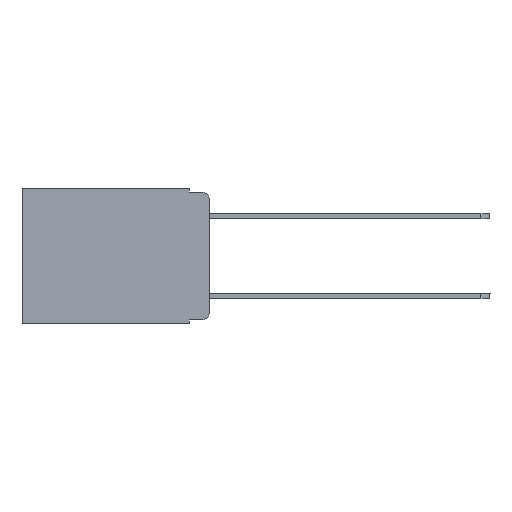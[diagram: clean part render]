
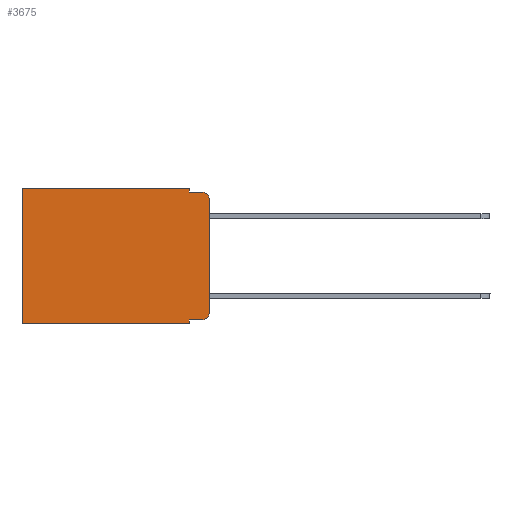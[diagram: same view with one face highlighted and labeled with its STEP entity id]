
A CAD part, left-side view. The second image highlights one B-rep face of the part: STEP entity #3675.
In plain terms, the highlighted planar face has unit normal (-1, 0, 0).
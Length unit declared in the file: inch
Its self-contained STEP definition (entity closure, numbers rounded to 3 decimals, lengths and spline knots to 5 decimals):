
#156 = EDGE_CURVE ( 'NONE', #4196, #10842, #6852, .T. ) ;
#284 = ORIENTED_EDGE ( 'NONE', *, *, #156, .T. ) ;
#360 = ORIENTED_EDGE ( 'NONE', *, *, #9546, .F. ) ;
#368 = VECTOR ( 'NONE', #1976, 39.37008 ) ;
#639 = DIRECTION ( 'NONE',  ( 0., -1., 0. ) ) ;
#705 = CARTESIAN_POINT ( 'NONE',  ( 0.298, 0., -0.03 ) ) ;
#710 = EDGE_CURVE ( 'NONE', #13267, #7853, #1727, .T. ) ;
#853 = VERTEX_POINT ( 'NONE', #5528 ) ;
#1153 = CARTESIAN_POINT ( 'NONE',  ( 0.298, 0.473, -0.343 ) ) ;
#1529 = VECTOR ( 'NONE', #7250, 39.37008 ) ;
#1727 = LINE ( 'NONE', #10578, #11859 ) ;
#1976 = DIRECTION ( 'NONE',  ( 0., 1., 0. ) ) ;
#2025 = CIRCLE ( 'NONE', #10658, 0.02 ) ;
#2625 = VERTEX_POINT ( 'NONE', #4624 ) ;
#2650 = CARTESIAN_POINT ( 'NONE',  ( 0.298, 0.02, -0.01 ) ) ;
#2816 = LINE ( 'NONE', #3873, #1529 ) ;
#2845 = DIRECTION ( 'NONE',  ( 0., 0., -1. ) ) ;
#2899 = DIRECTION ( 'NONE',  ( 0., 0., -1. ) ) ;
#2905 = CARTESIAN_POINT ( 'NONE',  ( 0.298, 0.051, -0.333 ) ) ;
#3022 = EDGE_CURVE ( 'NONE', #13267, #6196, #7514, .T. ) ;
#3092 = DIRECTION ( 'NONE',  ( -1., 0., 0. ) ) ;
#3662 = LINE ( 'NONE', #9221, #3977 ) ;
#3675 = ADVANCED_FACE ( 'NONE', ( #10889 ), #4963, .F. ) ;
#3873 = CARTESIAN_POINT ( 'NONE',  ( 0.298, 0.051, 0. ) ) ;
#3977 = VECTOR ( 'NONE', #13740, 39.37008 ) ;
#3985 = CARTESIAN_POINT ( 'NONE',  ( 0.298, 0., 0. ) ) ;
#4196 = VERTEX_POINT ( 'NONE', #2905 ) ;
#4624 = CARTESIAN_POINT ( 'NONE',  ( 0.298, 0.473, 0. ) ) ;
#4755 = ORIENTED_EDGE ( 'NONE', *, *, #3022, .T. ) ;
#4932 = LINE ( 'NONE', #9744, #6696 ) ;
#4963 = PLANE ( 'NONE',  #10207 ) ;
#5211 = ORIENTED_EDGE ( 'NONE', *, *, #12667, .F. ) ;
#5528 = CARTESIAN_POINT ( 'NONE',  ( 0.298, 0.051, -0.343 ) ) ;
#5583 = VECTOR ( 'NONE', #639, 39.37008 ) ;
#5769 = EDGE_CURVE ( 'NONE', #4196, #853, #2816, .T. ) ;
#6191 = DIRECTION ( 'NONE',  ( -1., 0., 0. ) ) ;
#6196 = VERTEX_POINT ( 'NONE', #2650 ) ;
#6286 = ORIENTED_EDGE ( 'NONE', *, *, #8117, .T. ) ;
#6696 = VECTOR ( 'NONE', #11826, 39.37008 ) ;
#6750 = ORIENTED_EDGE ( 'NONE', *, *, #8393, .F. ) ;
#6852 = LINE ( 'NONE', #14314, #5583 ) ;
#7104 = VERTEX_POINT ( 'NONE', #7624 ) ;
#7137 = CARTESIAN_POINT ( 'NONE',  ( 0.298, 0.051, -0.01 ) ) ;
#7218 = DIRECTION ( 'NONE',  ( 0., 0., -1. ) ) ;
#7250 = DIRECTION ( 'NONE',  ( 0., 0., -1. ) ) ;
#7295 = DIRECTION ( 'NONE',  ( 0., 0., -1. ) ) ;
#7348 = CARTESIAN_POINT ( 'NONE',  ( 0.298, 0.051, 0. ) ) ;
#7514 = CIRCLE ( 'NONE', #8480, 0.02 ) ;
#7533 = ORIENTED_EDGE ( 'NONE', *, *, #710, .F. ) ;
#7624 = CARTESIAN_POINT ( 'NONE',  ( 0.298, 0.051, 0. ) ) ;
#7853 = VERTEX_POINT ( 'NONE', #14838 ) ;
#8117 = EDGE_CURVE ( 'NONE', #10842, #7853, #2025, .T. ) ;
#8153 = EDGE_LOOP ( 'NONE', ( #7533, #4755, #5211, #360, #10105, #10697, #6750, #8561, #284, #6286 ) ) ;
#8393 = EDGE_CURVE ( 'NONE', #853, #12594, #14820, .T. ) ;
#8445 = EDGE_CURVE ( 'NONE', #2625, #12594, #10670, .T. ) ;
#8480 = AXIS2_PLACEMENT_3D ( 'NONE', #10080, #3092, #12251 ) ;
#8561 = ORIENTED_EDGE ( 'NONE', *, *, #5769, .F. ) ;
#9221 = CARTESIAN_POINT ( 'NONE',  ( 0.298, 0., 0. ) ) ;
#9419 = EDGE_CURVE ( 'NONE', #7104, #2625, #3662, .T. ) ;
#9546 = EDGE_CURVE ( 'NONE', #7104, #10195, #14400, .T. ) ;
#9730 = CARTESIAN_POINT ( 'NONE',  ( 0.298, 0.02, -0.313 ) ) ;
#9744 = CARTESIAN_POINT ( 'NONE',  ( 0.298, 0.051, -0.01 ) ) ;
#10080 = CARTESIAN_POINT ( 'NONE',  ( 0.298, 0.02, -0.03 ) ) ;
#10105 = ORIENTED_EDGE ( 'NONE', *, *, #9419, .T. ) ;
#10195 = VERTEX_POINT ( 'NONE', #7137 ) ;
#10207 = AXIS2_PLACEMENT_3D ( 'NONE', #3985, #13086, #2845 ) ;
#10224 = CARTESIAN_POINT ( 'NONE',  ( 0.298, 0., -0.343 ) ) ;
#10578 = CARTESIAN_POINT ( 'NONE',  ( 0.298, 0., 0. ) ) ;
#10588 = CARTESIAN_POINT ( 'NONE',  ( 0.298, 0.473, 0. ) ) ;
#10658 = AXIS2_PLACEMENT_3D ( 'NONE', #9730, #6191, #13400 ) ;
#10670 = LINE ( 'NONE', #10588, #12095 ) ;
#10697 = ORIENTED_EDGE ( 'NONE', *, *, #8445, .T. ) ;
#10718 = CARTESIAN_POINT ( 'NONE',  ( 0.298, 0.02, -0.333 ) ) ;
#10842 = VERTEX_POINT ( 'NONE', #10718 ) ;
#10889 = FACE_OUTER_BOUND ( 'NONE', #8153, .T. ) ;
#11826 = DIRECTION ( 'NONE',  ( 0., -1., 0. ) ) ;
#11859 = VECTOR ( 'NONE', #7295, 39.37008 ) ;
#12095 = VECTOR ( 'NONE', #7218, 39.37008 ) ;
#12251 = DIRECTION ( 'NONE',  ( 0., 0., -1. ) ) ;
#12594 = VERTEX_POINT ( 'NONE', #1153 ) ;
#12667 = EDGE_CURVE ( 'NONE', #10195, #6196, #4932, .T. ) ;
#13086 = DIRECTION ( 'NONE',  ( 1., 0., 0. ) ) ;
#13267 = VERTEX_POINT ( 'NONE', #705 ) ;
#13400 = DIRECTION ( 'NONE',  ( 0., 0., -1. ) ) ;
#13740 = DIRECTION ( 'NONE',  ( 0., 1., 0. ) ) ;
#14314 = CARTESIAN_POINT ( 'NONE',  ( 0.298, 0.051, -0.333 ) ) ;
#14400 = LINE ( 'NONE', #7348, #14553 ) ;
#14553 = VECTOR ( 'NONE', #2899, 39.37008 ) ;
#14820 = LINE ( 'NONE', #10224, #368 ) ;
#14838 = CARTESIAN_POINT ( 'NONE',  ( 0.298, 0., -0.313 ) ) ;
